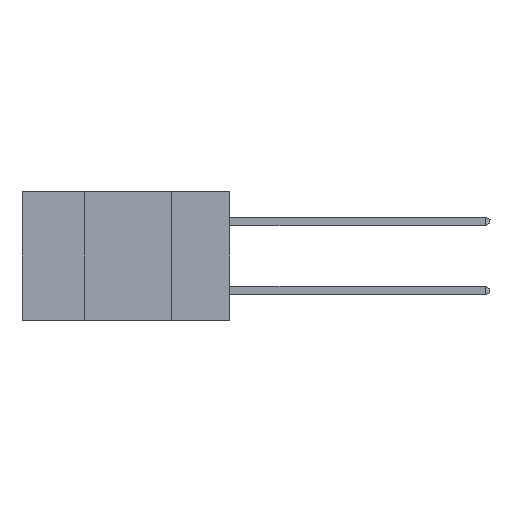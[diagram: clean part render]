
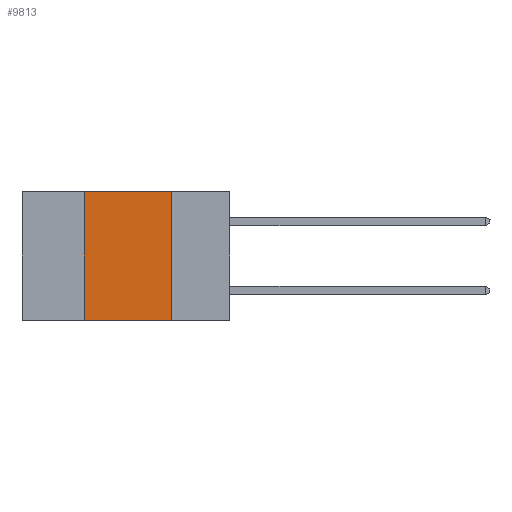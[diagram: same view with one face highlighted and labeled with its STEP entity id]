
A CAD part, left-side view. The second image highlights one B-rep face of the part: STEP entity #9813.
In plain terms, the highlighted planar face has unit normal (-1, 0, 0).
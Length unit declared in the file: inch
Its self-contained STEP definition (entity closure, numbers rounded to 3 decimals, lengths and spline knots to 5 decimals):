
#1490 = CARTESIAN_POINT ( 'NONE',  ( 0., 0.42, -0.37 ) ) ;
#1534 = CARTESIAN_POINT ( 'NONE',  ( 0., 0.6, 0. ) ) ;
#2326 = VECTOR ( 'NONE', #14784, 39.37008 ) ;
#2812 = DIRECTION ( 'NONE',  ( 0., 0., -1. ) ) ;
#3726 = CARTESIAN_POINT ( 'NONE',  ( 0., 0.6, 0. ) ) ;
#4144 = CARTESIAN_POINT ( 'NONE',  ( 0., 0.6, -0.37 ) ) ;
#4833 = PLANE ( 'NONE',  #9515 ) ;
#5673 = VECTOR ( 'NONE', #2812, 39.37008 ) ;
#5720 = VERTEX_POINT ( 'NONE', #8889 ) ;
#7343 = LINE ( 'NONE', #19252, #5673 ) ;
#7828 = EDGE_CURVE ( 'NONE', #19396, #10593, #8643, .T. ) ;
#7841 = CARTESIAN_POINT ( 'NONE',  ( 0., 0.42, -0.37 ) ) ;
#8643 = LINE ( 'NONE', #4144, #9410 ) ;
#8889 = CARTESIAN_POINT ( 'NONE',  ( 0., 0.17, 0. ) ) ;
#9094 = CARTESIAN_POINT ( 'NONE',  ( 0., 0.17, -0.37 ) ) ;
#9410 = VECTOR ( 'NONE', #10446, 39.37008 ) ;
#9515 = AXIS2_PLACEMENT_3D ( 'NONE', #3726, #16021, #11054 ) ;
#9813 = ADVANCED_FACE ( 'NONE', ( #18569 ), #4833, .F. ) ;
#9864 = VECTOR ( 'NONE', #13938, 39.37008 ) ;
#10095 = EDGE_CURVE ( 'NONE', #5720, #10593, #7343, .T. ) ;
#10446 = DIRECTION ( 'NONE',  ( 0., -1., 0. ) ) ;
#10526 = LINE ( 'NONE', #7841, #9864 ) ;
#10545 = VERTEX_POINT ( 'NONE', #19135 ) ;
#10593 = VERTEX_POINT ( 'NONE', #9094 ) ;
#11054 = DIRECTION ( 'NONE',  ( 0., 0., -1. ) ) ;
#11070 = ORIENTED_EDGE ( 'NONE', *, *, #7828, .T. ) ;
#11289 = ORIENTED_EDGE ( 'NONE', *, *, #11423, .F. ) ;
#11423 = EDGE_CURVE ( 'NONE', #19396, #10545, #10526, .T. ) ;
#13663 = ORIENTED_EDGE ( 'NONE', *, *, #10095, .F. ) ;
#13938 = DIRECTION ( 'NONE',  ( 0., 0., 1. ) ) ;
#14677 = LINE ( 'NONE', #1534, #2326 ) ;
#14784 = DIRECTION ( 'NONE',  ( 0., -1., 0. ) ) ;
#15223 = EDGE_LOOP ( 'NONE', ( #13663, #15350, #11289, #11070 ) ) ;
#15350 = ORIENTED_EDGE ( 'NONE', *, *, #18458, .F. ) ;
#16021 = DIRECTION ( 'NONE',  ( 1., 0., 0. ) ) ;
#18458 = EDGE_CURVE ( 'NONE', #10545, #5720, #14677, .T. ) ;
#18569 = FACE_OUTER_BOUND ( 'NONE', #15223, .T. ) ;
#19135 = CARTESIAN_POINT ( 'NONE',  ( 0., 0.42, 0. ) ) ;
#19252 = CARTESIAN_POINT ( 'NONE',  ( 0., 0.17, -0.37 ) ) ;
#19396 = VERTEX_POINT ( 'NONE', #1490 ) ;
